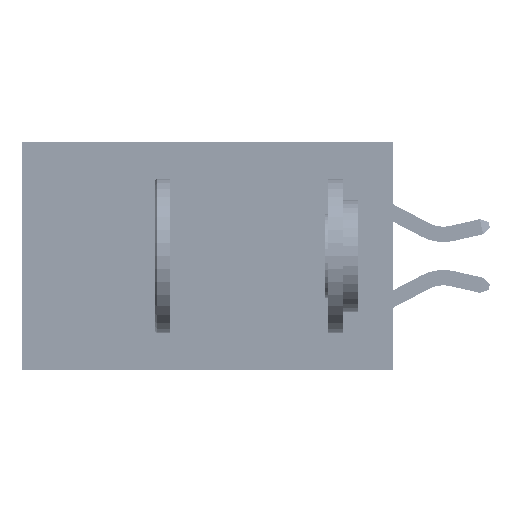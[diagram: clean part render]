
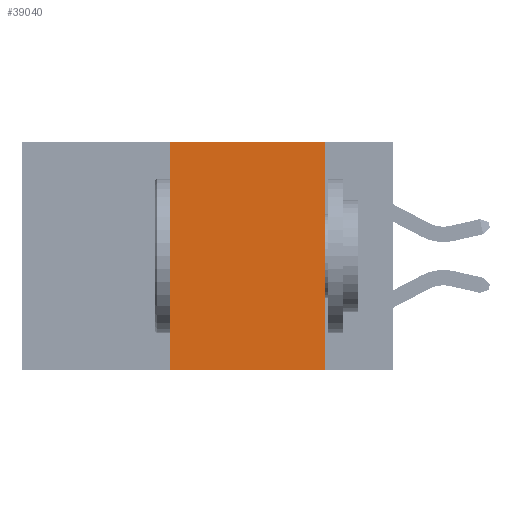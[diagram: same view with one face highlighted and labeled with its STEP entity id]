
A CAD part, left-side view. The second image highlights one B-rep face of the part: STEP entity #39040.
In plain terms, the highlighted planar face has unit normal (-1, 0, 0).
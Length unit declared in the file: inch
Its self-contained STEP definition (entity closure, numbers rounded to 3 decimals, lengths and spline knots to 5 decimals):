
#27 = DIRECTION ( 'NONE',  ( 0., 0., -1. ) ) ;
#1320 = DIRECTION ( 'NONE',  ( 0., 0., -1. ) ) ;
#1764 = VECTOR ( 'NONE', #27, 39.37008 ) ;
#3253 = CARTESIAN_POINT ( 'NONE',  ( 0., 0.11, 0. ) ) ;
#5816 = LINE ( 'NONE', #32191, #33161 ) ;
#9732 = EDGE_CURVE ( 'NONE', #25278, #20225, #39806, .T. ) ;
#10025 = EDGE_LOOP ( 'NONE', ( #13328, #39970, #32831, #46006 ) ) ;
#10615 = CARTESIAN_POINT ( 'NONE',  ( 0., 0.36, 0. ) ) ;
#12648 = EDGE_CURVE ( 'NONE', #14983, #25278, #23512, .T. ) ;
#13328 = ORIENTED_EDGE ( 'NONE', *, *, #9732, .F. ) ;
#14983 = VERTEX_POINT ( 'NONE', #10615 ) ;
#15503 = EDGE_CURVE ( 'NONE', #42718, #20225, #16408, .T. ) ;
#16408 = LINE ( 'NONE', #17026, #43499 ) ;
#17026 = CARTESIAN_POINT ( 'NONE',  ( 0., 0.6, -0.37 ) ) ;
#17324 = CARTESIAN_POINT ( 'NONE',  ( 0., 0.6, 0. ) ) ;
#19443 = PLANE ( 'NONE',  #25167 ) ;
#20225 = VERTEX_POINT ( 'NONE', #25133 ) ;
#20601 = DIRECTION ( 'NONE',  ( 0., -1., 0. ) ) ;
#22296 = CARTESIAN_POINT ( 'NONE',  ( 0., 0.36, -0.37 ) ) ;
#22989 = DIRECTION ( 'NONE',  ( 1., 0., 0. ) ) ;
#23512 = LINE ( 'NONE', #17324, #43406 ) ;
#25133 = CARTESIAN_POINT ( 'NONE',  ( 0., 0.11, -0.37 ) ) ;
#25167 = AXIS2_PLACEMENT_3D ( 'NONE', #44154, #22989, #1320 ) ;
#25278 = VERTEX_POINT ( 'NONE', #3253 ) ;
#32191 = CARTESIAN_POINT ( 'NONE',  ( 0., 0.36, 0. ) ) ;
#32831 = ORIENTED_EDGE ( 'NONE', *, *, #46318, .F. ) ;
#33161 = VECTOR ( 'NONE', #35773, 39.37008 ) ;
#35773 = DIRECTION ( 'NONE',  ( 0., 0., 1. ) ) ;
#38852 = FACE_OUTER_BOUND ( 'NONE', #10025, .T. ) ;
#39040 = ADVANCED_FACE ( 'NONE', ( #38852 ), #19443, .F. ) ;
#39538 = CARTESIAN_POINT ( 'NONE',  ( 0., 0.11, 0. ) ) ;
#39806 = LINE ( 'NONE', #39538, #1764 ) ;
#39970 = ORIENTED_EDGE ( 'NONE', *, *, #12648, .F. ) ;
#42718 = VERTEX_POINT ( 'NONE', #22296 ) ;
#43406 = VECTOR ( 'NONE', #45602, 39.37008 ) ;
#43499 = VECTOR ( 'NONE', #20601, 39.37008 ) ;
#44154 = CARTESIAN_POINT ( 'NONE',  ( 0., 0.6, 0. ) ) ;
#45602 = DIRECTION ( 'NONE',  ( 0., -1., 0. ) ) ;
#46006 = ORIENTED_EDGE ( 'NONE', *, *, #15503, .T. ) ;
#46318 = EDGE_CURVE ( 'NONE', #42718, #14983, #5816, .T. ) ;
